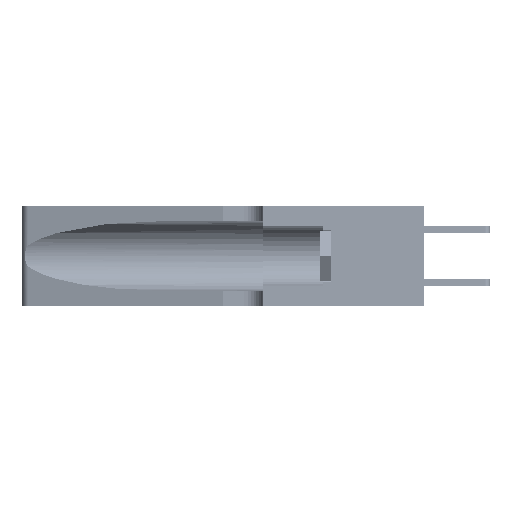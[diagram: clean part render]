
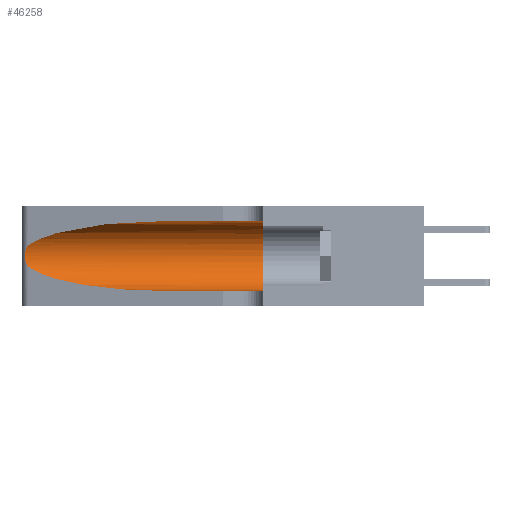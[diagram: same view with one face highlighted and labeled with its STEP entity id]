
A CAD part, left-side view. The second image highlights one B-rep face of the part: STEP entity #46258.
In plain terms, the highlighted cylindrical face has radius 3.308 mm (diameter 6.617 mm), a partial arc.
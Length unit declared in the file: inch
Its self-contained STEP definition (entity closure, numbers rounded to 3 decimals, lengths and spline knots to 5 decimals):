
#268 =( BOUNDED_CURVE ( )  B_SPLINE_CURVE ( 3, ( #11999, #44674, #30216, #22421 ),
 .UNSPECIFIED., .F., .F. ) 
 B_SPLINE_CURVE_WITH_KNOTS ( ( 4, 4 ),
 ( 1.5708, 2.84003 ),
 .UNSPECIFIED. ) 
 CURVE ( )  GEOMETRIC_REPRESENTATION_ITEM ( )  RATIONAL_B_SPLINE_CURVE ( ( 1., 0.87, 0.87, 1. ) ) 
 REPRESENTATION_ITEM ( '' )  );
#399 = LINE ( 'NONE', #33505, #1582 ) ;
#1072 = CARTESIAN_POINT ( 'NONE',  ( 0.26017, 1.23833, 0.17102 ) ) ;
#1582 = VECTOR ( 'NONE', #4949, 39.37008 ) ;
#3055 = EDGE_CURVE ( 'NONE', #34205, #24318, #399, .T. ) ;
#3083 = EDGE_CURVE ( 'NONE', #44299, #21492, #22604, .T. ) ;
#4314 = DIRECTION ( 'NONE',  ( 0., 1., 0. ) ) ;
#4389 = DIRECTION ( 'NONE',  ( 0., -1., 0. ) ) ;
#4796 = CARTESIAN_POINT ( 'NONE',  ( 0.25487, 1.22718, 0.14631 ) ) ;
#4949 = DIRECTION ( 'NONE',  ( 0., -1., 0. ) ) ;
#5349 = FACE_OUTER_BOUND ( 'NONE', #23049, .T. ) ;
#7769 = EDGE_CURVE ( 'NONE', #21492, #9549, #17521, .T. ) ;
#8066 = AXIS2_PLACEMENT_3D ( 'NONE', #26625, #4389, #33916 ) ;
#8663 = CARTESIAN_POINT ( 'NONE',  ( 0.25487, 1.22718, 0.22369 ) ) ;
#8822 = CARTESIAN_POINT ( 'NONE',  ( 0.25787, 1.23484, 0.2124 ) ) ;
#9549 = VERTEX_POINT ( 'NONE', #37903 ) ;
#11338 = ORIENTED_EDGE ( 'NONE', *, *, #3083, .T. ) ;
#11402 = CARTESIAN_POINT ( 'NONE',  ( 0.1305, 0.35, 0.05475 ) ) ;
#11523 = AXIS2_PLACEMENT_3D ( 'NONE', #30130, #4314, #30297 ) ;
#11623 = CARTESIAN_POINT ( 'NONE',  ( 0.1305, 0.72297, 0.31525 ) ) ;
#11795 = LINE ( 'NONE', #46857, #18767 ) ;
#11999 = CARTESIAN_POINT ( 'NONE',  ( 0.1305, 0.72297, 0.31525 ) ) ;
#12019 = ORIENTED_EDGE ( 'NONE', *, *, #3055, .F. ) ;
#12045 = CARTESIAN_POINT ( 'NONE',  ( 0.1305, 0.35, 0.31525 ) ) ;
#14765 = EDGE_CURVE ( 'NONE', #34205, #44299, #268, .T. ) ;
#15809 = CARTESIAN_POINT ( 'NONE',  ( 0.26075, 1.23896, 0.178 ) ) ;
#17521 =( BOUNDED_CURVE ( )  B_SPLINE_CURVE ( 3, ( #30850, #43976, #29337, #47668 ),
 .UNSPECIFIED., .F., .F. ) 
 B_SPLINE_CURVE_WITH_KNOTS ( ( 4, 4 ),
 ( 3.44316, 4.71239 ),
 .UNSPECIFIED. ) 
 CURVE ( )  GEOMETRIC_REPRESENTATION_ITEM ( )  RATIONAL_B_SPLINE_CURVE ( ( 1., 0.87, 0.87, 1. ) ) 
 REPRESENTATION_ITEM ( '' )  );
#18767 = VECTOR ( 'NONE', #28521, 39.37008 ) ;
#20022 = CARTESIAN_POINT ( 'NONE',  ( 0.25789, 1.23486, 0.15765 ) ) ;
#21492 = VERTEX_POINT ( 'NONE', #48055 ) ;
#22421 = CARTESIAN_POINT ( 'NONE',  ( 0.25487, 1.22718, 0.22369 ) ) ;
#22448 = ORIENTED_EDGE ( 'NONE', *, *, #14765, .T. ) ;
#22604 = B_SPLINE_CURVE_WITH_KNOTS ( 'NONE', 3,
 ( #8663, #23320, #23480, #8822, #38075, #23632, #27355, #15809, #1072, #27036, #20022, #34633, #23785, #4796 ),
 .UNSPECIFIED., .F., .F.,
 ( 4, 2, 2, 2, 2, 2, 4 ),
 ( 0., 0.00027, 0.00053, 0.00107, 0.0016, 0.00187, 0.00214 ),
 .UNSPECIFIED. ) ;
#23049 = EDGE_LOOP ( 'NONE', ( #22448, #11338, #40263, #48043, #25313, #12019 ) ) ;
#23320 = CARTESIAN_POINT ( 'NONE',  ( 0.25555, 1.22994, 0.2215 ) ) ;
#23480 = CARTESIAN_POINT ( 'NONE',  ( 0.25639, 1.23184, 0.21858 ) ) ;
#23632 = CARTESIAN_POINT ( 'NONE',  ( 0.26018, 1.23835, 0.19895 ) ) ;
#23785 = CARTESIAN_POINT ( 'NONE',  ( 0.25555, 1.22993, 0.14849 ) ) ;
#24318 = VERTEX_POINT ( 'NONE', #12045 ) ;
#25313 = ORIENTED_EDGE ( 'NONE', *, *, #29895, .F. ) ;
#26625 = CARTESIAN_POINT ( 'NONE',  ( 0.1305, 1.61858, 0.185 ) ) ;
#27036 = CARTESIAN_POINT ( 'NONE',  ( 0.25856, 1.23593, 0.16098 ) ) ;
#27355 = CARTESIAN_POINT ( 'NONE',  ( 0.26075, 1.23896, 0.19203 ) ) ;
#28521 = DIRECTION ( 'NONE',  ( 0., -1., 0. ) ) ;
#29337 = CARTESIAN_POINT ( 'NONE',  ( 0.18966, 0.96281, 0.05475 ) ) ;
#29895 = EDGE_CURVE ( 'NONE', #24318, #37558, #34697, .T. ) ;
#30130 = CARTESIAN_POINT ( 'NONE',  ( 0.1305, 0.35, 0.185 ) ) ;
#30216 = CARTESIAN_POINT ( 'NONE',  ( 0.2373, 1.15595, 0.28018 ) ) ;
#30297 = DIRECTION ( 'NONE',  ( 0., 0., 1. ) ) ;
#30850 = CARTESIAN_POINT ( 'NONE',  ( 0.25487, 1.22718, 0.14631 ) ) ;
#33505 = CARTESIAN_POINT ( 'NONE',  ( 0.1305, 1.61858, 0.31525 ) ) ;
#33916 = DIRECTION ( 'NONE',  ( 0., 0., -1. ) ) ;
#34205 = VERTEX_POINT ( 'NONE', #11623 ) ;
#34399 = EDGE_CURVE ( 'NONE', #9549, #37558, #11795, .T. ) ;
#34633 = CARTESIAN_POINT ( 'NONE',  ( 0.25639, 1.23186, 0.15144 ) ) ;
#34697 = CIRCLE ( 'NONE', #11523, 0.13025 ) ;
#37288 = CYLINDRICAL_SURFACE ( 'NONE', #8066, 0.13025 ) ;
#37558 = VERTEX_POINT ( 'NONE', #11402 ) ;
#37903 = CARTESIAN_POINT ( 'NONE',  ( 0.1305, 0.72297, 0.05475 ) ) ;
#38075 = CARTESIAN_POINT ( 'NONE',  ( 0.25854, 1.2359, 0.20912 ) ) ;
#39416 = CARTESIAN_POINT ( 'NONE',  ( 0.25487, 1.22718, 0.22369 ) ) ;
#40263 = ORIENTED_EDGE ( 'NONE', *, *, #7769, .T. ) ;
#43976 = CARTESIAN_POINT ( 'NONE',  ( 0.2373, 1.15595, 0.08982 ) ) ;
#44299 = VERTEX_POINT ( 'NONE', #39416 ) ;
#44674 = CARTESIAN_POINT ( 'NONE',  ( 0.18966, 0.96281, 0.31525 ) ) ;
#46258 = ADVANCED_FACE ( 'NONE', ( #5349 ), #37288, .F. ) ;
#46857 = CARTESIAN_POINT ( 'NONE',  ( 0.1305, 1.61858, 0.05475 ) ) ;
#47668 = CARTESIAN_POINT ( 'NONE',  ( 0.1305, 0.72297, 0.05475 ) ) ;
#48043 = ORIENTED_EDGE ( 'NONE', *, *, #34399, .T. ) ;
#48055 = CARTESIAN_POINT ( 'NONE',  ( 0.25487, 1.22718, 0.14631 ) ) ;
